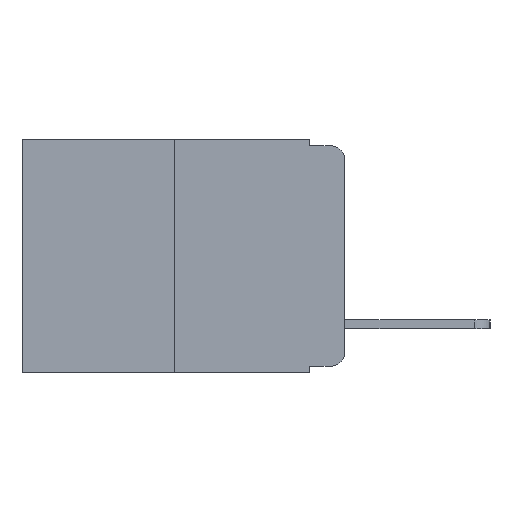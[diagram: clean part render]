
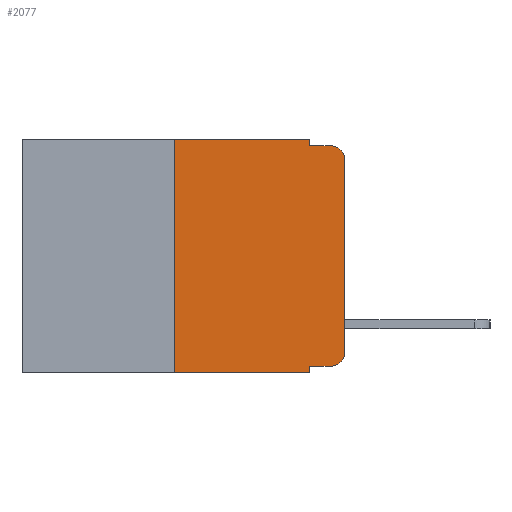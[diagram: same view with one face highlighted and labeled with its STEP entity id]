
A CAD part, left-side view. The second image highlights one B-rep face of the part: STEP entity #2077.
In plain terms, the highlighted planar face has unit normal (-1, 0, 0).
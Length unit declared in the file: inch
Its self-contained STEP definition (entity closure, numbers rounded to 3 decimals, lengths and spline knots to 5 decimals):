
#60 = VERTEX_POINT ( 'NONE', #10239 ) ;
#337 = VECTOR ( 'NONE', #1821, 39.37008 ) ;
#433 = CARTESIAN_POINT ( 'NONE',  ( 0., 0.051, 0. ) ) ;
#539 = DIRECTION ( 'NONE',  ( 0., -1., 0. ) ) ;
#599 = DIRECTION ( 'NONE',  ( 0., 0., -1. ) ) ;
#663 = ORIENTED_EDGE ( 'NONE', *, *, #12895, .F. ) ;
#691 = ORIENTED_EDGE ( 'NONE', *, *, #12877, .F. ) ;
#744 = CIRCLE ( 'NONE', #12920, 0.02 ) ;
#811 = ORIENTED_EDGE ( 'NONE', *, *, #12942, .T. ) ;
#913 = DIRECTION ( 'NONE',  ( 0., 0., -1. ) ) ;
#1139 = VECTOR ( 'NONE', #7024, 39.37008 ) ;
#1143 = VERTEX_POINT ( 'NONE', #10858 ) ;
#1439 = ORIENTED_EDGE ( 'NONE', *, *, #4322, .F. ) ;
#1730 = CARTESIAN_POINT ( 'NONE',  ( 0., 0.051, 0. ) ) ;
#1821 = DIRECTION ( 'NONE',  ( 0., 0., 1. ) ) ;
#2077 = ADVANCED_FACE ( 'NONE', ( #8857 ), #3152, .F. ) ;
#2195 = ORIENTED_EDGE ( 'NONE', *, *, #12398, .T. ) ;
#2374 = VECTOR ( 'NONE', #9050, 39.37008 ) ;
#2381 = LINE ( 'NONE', #3204, #7588 ) ;
#2510 = ORIENTED_EDGE ( 'NONE', *, *, #12880, .F. ) ;
#2589 = CARTESIAN_POINT ( 'NONE',  ( 0., 0., -0.03 ) ) ;
#2767 = ORIENTED_EDGE ( 'NONE', *, *, #12927, .T. ) ;
#2879 = CARTESIAN_POINT ( 'NONE',  ( 0., 0.051, -0.01 ) ) ;
#3020 = VECTOR ( 'NONE', #11369, 39.37008 ) ;
#3108 = CARTESIAN_POINT ( 'NONE',  ( 0., 0.25, 0. ) ) ;
#3148 = DIRECTION ( 'NONE',  ( 0., -1., 0. ) ) ;
#3152 = PLANE ( 'NONE',  #4946 ) ;
#3204 = CARTESIAN_POINT ( 'NONE',  ( 0., 0.473, -0.343 ) ) ;
#3367 = LINE ( 'NONE', #6056, #337 ) ;
#3459 = CARTESIAN_POINT ( 'NONE',  ( 0., 0.473, 0. ) ) ;
#3566 = CARTESIAN_POINT ( 'NONE',  ( 0., 0.051, -0.333 ) ) ;
#3714 = VECTOR ( 'NONE', #539, 39.37008 ) ;
#3889 = VERTEX_POINT ( 'NONE', #3566 ) ;
#3894 = VERTEX_POINT ( 'NONE', #2879 ) ;
#3917 = CARTESIAN_POINT ( 'NONE',  ( 0., 0.25, 0. ) ) ;
#4104 = LINE ( 'NONE', #7940, #1139 ) ;
#4216 = DIRECTION ( 'NONE',  ( 1., 0., 0. ) ) ;
#4322 = EDGE_CURVE ( 'NONE', #12330, #6399, #10935, .T. ) ;
#4446 = AXIS2_PLACEMENT_3D ( 'NONE', #11456, #5805, #12412 ) ;
#4491 = LINE ( 'NONE', #433, #6796 ) ;
#4695 = ORIENTED_EDGE ( 'NONE', *, *, #13013, .T. ) ;
#4888 = ORIENTED_EDGE ( 'NONE', *, *, #13069, .T. ) ;
#4946 = AXIS2_PLACEMENT_3D ( 'NONE', #10241, #4216, #913 ) ;
#5338 = VERTEX_POINT ( 'NONE', #8089 ) ;
#5625 = ORIENTED_EDGE ( 'NONE', *, *, #12866, .F. ) ;
#5805 = DIRECTION ( 'NONE',  ( -1., 0., 0. ) ) ;
#6013 = CARTESIAN_POINT ( 'NONE',  ( 0., 0.051, -0.01 ) ) ;
#6056 = CARTESIAN_POINT ( 'NONE',  ( 0., 0., 0. ) ) ;
#6387 = VERTEX_POINT ( 'NONE', #10641 ) ;
#6399 = VERTEX_POINT ( 'NONE', #1730 ) ;
#6796 = VECTOR ( 'NONE', #6976, 39.37008 ) ;
#6976 = DIRECTION ( 'NONE',  ( 0., 0., -1. ) ) ;
#7024 = DIRECTION ( 'NONE',  ( 0., 0., -1. ) ) ;
#7068 = DIRECTION ( 'NONE',  ( -1., 0., 0. ) ) ;
#7588 = VECTOR ( 'NONE', #3148, 39.37008 ) ;
#7940 = CARTESIAN_POINT ( 'NONE',  ( 0., 0.051, 0. ) ) ;
#8089 = CARTESIAN_POINT ( 'NONE',  ( 0., 0.25, -0.343 ) ) ;
#8108 = CARTESIAN_POINT ( 'NONE',  ( 0., 0.051, -0.333 ) ) ;
#8857 = FACE_OUTER_BOUND ( 'NONE', #9041, .T. ) ;
#9041 = EDGE_LOOP ( 'NONE', ( #811, #2767, #663, #2510, #1439, #691, #2195, #5625, #4695, #4888 ) ) ;
#9050 = DIRECTION ( 'NONE',  ( 0., -1., 0. ) ) ;
#9342 = LINE ( 'NONE', #3917, #11502 ) ;
#10239 = CARTESIAN_POINT ( 'NONE',  ( 0., 0.02, -0.01 ) ) ;
#10241 = CARTESIAN_POINT ( 'NONE',  ( 0., 0.473, 0. ) ) ;
#10375 = LINE ( 'NONE', #8108, #2374 ) ;
#10641 = CARTESIAN_POINT ( 'NONE',  ( 0., 0.02, -0.333 ) ) ;
#10858 = CARTESIAN_POINT ( 'NONE',  ( 0., 0.051, -0.343 ) ) ;
#10935 = LINE ( 'NONE', #3459, #3020 ) ;
#11063 = VERTEX_POINT ( 'NONE', #2589 ) ;
#11123 = CARTESIAN_POINT ( 'NONE',  ( 0., 0., -0.313 ) ) ;
#11369 = DIRECTION ( 'NONE',  ( 0., -1., 0. ) ) ;
#11456 = CARTESIAN_POINT ( 'NONE',  ( 0., 0.02, -0.313 ) ) ;
#11502 = VECTOR ( 'NONE', #11661, 39.37008 ) ;
#11661 = DIRECTION ( 'NONE',  ( 0., 0., 1. ) ) ;
#11803 = LINE ( 'NONE', #6013, #3714 ) ;
#11938 = VERTEX_POINT ( 'NONE', #11123 ) ;
#11960 = CIRCLE ( 'NONE', #4446, 0.02 ) ;
#12330 = VERTEX_POINT ( 'NONE', #3108 ) ;
#12398 = EDGE_CURVE ( 'NONE', #5338, #1143, #2381, .T. ) ;
#12412 = DIRECTION ( 'NONE',  ( 0., 0., -1. ) ) ;
#12635 = CARTESIAN_POINT ( 'NONE',  ( 0., 0.02, -0.03 ) ) ;
#12866 = EDGE_CURVE ( 'NONE', #3889, #1143, #4491, .T. ) ;
#12877 = EDGE_CURVE ( 'NONE', #5338, #12330, #9342, .T. ) ;
#12880 = EDGE_CURVE ( 'NONE', #6399, #3894, #4104, .T. ) ;
#12895 = EDGE_CURVE ( 'NONE', #3894, #60, #11803, .T. ) ;
#12920 = AXIS2_PLACEMENT_3D ( 'NONE', #12635, #7068, #599 ) ;
#12927 = EDGE_CURVE ( 'NONE', #11063, #60, #744, .T. ) ;
#12942 = EDGE_CURVE ( 'NONE', #11938, #11063, #3367, .T. ) ;
#13013 = EDGE_CURVE ( 'NONE', #3889, #6387, #10375, .T. ) ;
#13069 = EDGE_CURVE ( 'NONE', #6387, #11938, #11960, .T. ) ;
